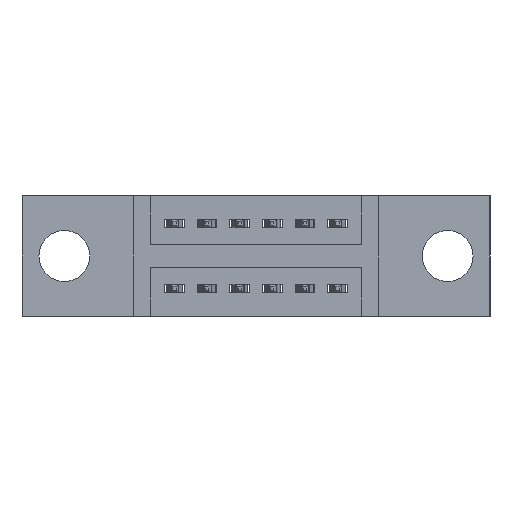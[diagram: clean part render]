
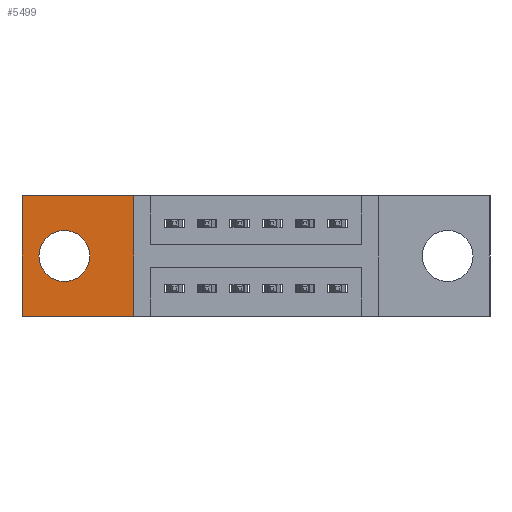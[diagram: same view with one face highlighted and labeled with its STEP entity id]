
A CAD part, front view. The second image highlights one B-rep face of the part: STEP entity #5499.
In plain terms, the highlighted planar face has unit normal (0, -1, 0).
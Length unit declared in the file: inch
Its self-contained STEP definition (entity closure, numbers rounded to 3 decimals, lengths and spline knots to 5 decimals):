
#83 = CARTESIAN_POINT ( 'NONE',  ( 0., 0.11, 0. ) ) ;
#193 = CARTESIAN_POINT ( 'NONE',  ( 0.3425, 0.11, -0.37 ) ) ;
#239 = VERTEX_POINT ( 'NONE', #193 ) ;
#316 = ORIENTED_EDGE ( 'NONE', *, *, #4395, .F. ) ;
#320 = DIRECTION ( 'NONE',  ( 1., 0., 0. ) ) ;
#565 = CARTESIAN_POINT ( 'NONE',  ( 0., 0.11, 0. ) ) ;
#771 = CARTESIAN_POINT ( 'NONE',  ( 0.13, 0.11, -0.263 ) ) ;
#861 = VERTEX_POINT ( 'NONE', #8908 ) ;
#985 = AXIS2_PLACEMENT_3D ( 'NONE', #8962, #8960, #8952 ) ;
#1231 = CARTESIAN_POINT ( 'NONE',  ( 0., 0.11, -0.37 ) ) ;
#1479 = ORIENTED_EDGE ( 'NONE', *, *, #7232, .T. ) ;
#1694 = CIRCLE ( 'NONE', #985, 0.078 ) ;
#1756 = VECTOR ( 'NONE', #3361, 39.37008 ) ;
#1974 = ORIENTED_EDGE ( 'NONE', *, *, #5743, .T. ) ;
#1980 = VERTEX_POINT ( 'NONE', #565 ) ;
#2050 = FACE_OUTER_BOUND ( 'NONE', #7102, .T. ) ;
#2282 = CARTESIAN_POINT ( 'NONE',  ( 0., 0.11, -0.37 ) ) ;
#3143 = CARTESIAN_POINT ( 'NONE',  ( 0., 0.11, 0. ) ) ;
#3343 = CIRCLE ( 'NONE', #6245, 0.078 ) ;
#3361 = DIRECTION ( 'NONE',  ( 0., 0., -1. ) ) ;
#3436 = CARTESIAN_POINT ( 'NONE',  ( 0.13, 0.11, -0.185 ) ) ;
#3600 = ORIENTED_EDGE ( 'NONE', *, *, #9172, .T. ) ;
#3904 = LINE ( 'NONE', #83, #1756 ) ;
#4306 = DIRECTION ( 'NONE',  ( 0., 0., -1. ) ) ;
#4395 = EDGE_CURVE ( 'NONE', #5203, #861, #1694, .T. ) ;
#4803 = DIRECTION ( 'NONE',  ( 0., -1., 0. ) ) ;
#5203 = VERTEX_POINT ( 'NONE', #771 ) ;
#5294 = CARTESIAN_POINT ( 'NONE',  ( 0.3425, 0.11, 0. ) ) ;
#5499 = ADVANCED_FACE ( 'NONE', ( #8190, #2050 ), #8984, .T. ) ;
#5550 = EDGE_LOOP ( 'NONE', ( #8329, #316 ) ) ;
#5743 = EDGE_CURVE ( 'NONE', #239, #6595, #7694, .T. ) ;
#6245 = AXIS2_PLACEMENT_3D ( 'NONE', #3436, #8651, #4306 ) ;
#6595 = VERTEX_POINT ( 'NONE', #9383 ) ;
#6645 = VECTOR ( 'NONE', #320, 39.37008 ) ;
#6687 = VERTEX_POINT ( 'NONE', #1231 ) ;
#6921 = LINE ( 'NONE', #3143, #8444 ) ;
#7046 = VECTOR ( 'NONE', #8106, 39.37008 ) ;
#7102 = EDGE_LOOP ( 'NONE', ( #1479, #3600, #1974, #9390 ) ) ;
#7232 = EDGE_CURVE ( 'NONE', #1980, #6687, #3904, .T. ) ;
#7694 = LINE ( 'NONE', #5294, #7046 ) ;
#7899 = EDGE_CURVE ( 'NONE', #6595, #1980, #6921, .T. ) ;
#8106 = DIRECTION ( 'NONE',  ( 0., 0., 1. ) ) ;
#8190 = FACE_BOUND ( 'NONE', #5550, .T. ) ;
#8329 = ORIENTED_EDGE ( 'NONE', *, *, #9046, .F. ) ;
#8410 = LINE ( 'NONE', #9321, #6645 ) ;
#8444 = VECTOR ( 'NONE', #9654, 39.37008 ) ;
#8651 = DIRECTION ( 'NONE',  ( 0., -1., 0. ) ) ;
#8908 = CARTESIAN_POINT ( 'NONE',  ( 0.13, 0.11, -0.107 ) ) ;
#8952 = DIRECTION ( 'NONE',  ( 0., 0., -1. ) ) ;
#8960 = DIRECTION ( 'NONE',  ( 0., -1., 0. ) ) ;
#8962 = CARTESIAN_POINT ( 'NONE',  ( 0.13, 0.11, -0.185 ) ) ;
#8984 = PLANE ( 'NONE',  #9255 ) ;
#9046 = EDGE_CURVE ( 'NONE', #861, #5203, #3343, .T. ) ;
#9172 = EDGE_CURVE ( 'NONE', #6687, #239, #8410, .T. ) ;
#9255 = AXIS2_PLACEMENT_3D ( 'NONE', #2282, #4803, #9604 ) ;
#9321 = CARTESIAN_POINT ( 'NONE',  ( 0., 0.11, -0.37 ) ) ;
#9383 = CARTESIAN_POINT ( 'NONE',  ( 0.3425, 0.11, 0. ) ) ;
#9390 = ORIENTED_EDGE ( 'NONE', *, *, #7899, .T. ) ;
#9604 = DIRECTION ( 'NONE',  ( 0., 0., -1. ) ) ;
#9654 = DIRECTION ( 'NONE',  ( -1., 0., 0. ) ) ;
